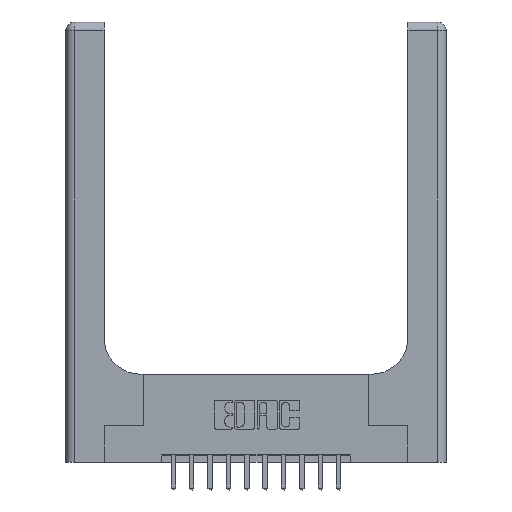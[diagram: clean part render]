
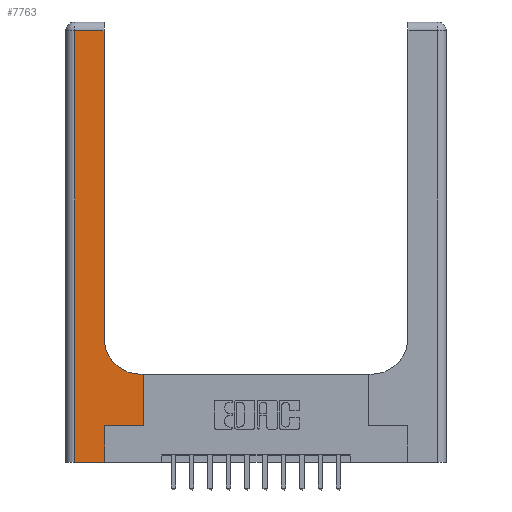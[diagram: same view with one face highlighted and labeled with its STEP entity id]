
A CAD part, top view. The second image highlights one B-rep face of the part: STEP entity #7763.
In plain terms, the highlighted planar face has unit normal (0, 0, 1).
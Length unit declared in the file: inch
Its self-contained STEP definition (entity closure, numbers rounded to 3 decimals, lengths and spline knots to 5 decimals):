
#154 = ORIENTED_EDGE ( 'NONE', *, *, #16225, .T. ) ;
#379 = EDGE_CURVE ( 'NONE', #7380, #3538, #15447, .T. ) ;
#570 = VECTOR ( 'NONE', #12872, 39.37008 ) ;
#576 = CARTESIAN_POINT ( 'NONE',  ( 0.26, 3., 0.37 ) ) ;
#1165 = VECTOR ( 'NONE', #13585, 39.37008 ) ;
#1371 = EDGE_CURVE ( 'NONE', #15486, #11015, #5670, .T. ) ;
#1570 = VERTEX_POINT ( 'NONE', #15523 ) ;
#1646 = DIRECTION ( 'NONE',  ( -1., 0., 0. ) ) ;
#1706 = VECTOR ( 'NONE', #1646, 39.37008 ) ;
#2901 = VERTEX_POINT ( 'NONE', #3424 ) ;
#3424 = CARTESIAN_POINT ( 'NONE',  ( 0.26, 0.85, 0.37 ) ) ;
#3435 = ORIENTED_EDGE ( 'NONE', *, *, #14333, .T. ) ;
#3538 = VERTEX_POINT ( 'NONE', #16037 ) ;
#3654 = CARTESIAN_POINT ( 'NONE',  ( 0.06, 0., 0.37 ) ) ;
#3705 = CARTESIAN_POINT ( 'NONE',  ( 0., 0., 0.37 ) ) ;
#3784 = EDGE_CURVE ( 'NONE', #2901, #15486, #15676, .T. ) ;
#3901 = DIRECTION ( 'NONE',  ( 1., 0., 0. ) ) ;
#4111 = VECTOR ( 'NONE', #7776, 39.37008 ) ;
#4135 = EDGE_CURVE ( 'NONE', #3538, #8264, #15314, .T. ) ;
#4285 = CARTESIAN_POINT ( 'NONE',  ( 0.26, 2.94, 0.37 ) ) ;
#4526 = ORIENTED_EDGE ( 'NONE', *, *, #379, .T. ) ;
#4615 = CARTESIAN_POINT ( 'NONE',  ( 0.51, 0.85, 0.37 ) ) ;
#4863 = AXIS2_PLACEMENT_3D ( 'NONE', #14027, #8760, #7678 ) ;
#5261 = PLANE ( 'NONE',  #4863 ) ;
#5432 = EDGE_CURVE ( 'NONE', #1570, #2901, #13335, .T. ) ;
#5670 = LINE ( 'NONE', #10921, #1165 ) ;
#7380 = VERTEX_POINT ( 'NONE', #12866 ) ;
#7503 = FACE_OUTER_BOUND ( 'NONE', #15960, .T. ) ;
#7634 = VECTOR ( 'NONE', #13767, 39.37008 ) ;
#7678 = DIRECTION ( 'NONE',  ( -1., 0., 0. ) ) ;
#7763 = ADVANCED_FACE ( 'NONE', ( #7503 ), #5261, .F. ) ;
#7776 = DIRECTION ( 'NONE',  ( 0., 1., 0. ) ) ;
#8211 = DIRECTION ( 'NONE',  ( 0., 1., 0. ) ) ;
#8264 = VERTEX_POINT ( 'NONE', #15177 ) ;
#8537 = AXIS2_PLACEMENT_3D ( 'NONE', #4615, #9543, #13474 ) ;
#8679 = LINE ( 'NONE', #10003, #7634 ) ;
#8732 = ORIENTED_EDGE ( 'NONE', *, *, #3784, .T. ) ;
#8760 = DIRECTION ( 'NONE',  ( 0., 0., -1. ) ) ;
#9213 = ORIENTED_EDGE ( 'NONE', *, *, #10492, .T. ) ;
#9543 = DIRECTION ( 'NONE',  ( 0., 0., -1. ) ) ;
#9678 = ORIENTED_EDGE ( 'NONE', *, *, #5432, .T. ) ;
#9757 = ORIENTED_EDGE ( 'NONE', *, *, #4135, .T. ) ;
#10003 = CARTESIAN_POINT ( 'NONE',  ( 0.06, 3., 0.37 ) ) ;
#10386 = ORIENTED_EDGE ( 'NONE', *, *, #14854, .T. ) ;
#10406 = CARTESIAN_POINT ( 'NONE',  ( 0.265, 0.25, 0.37 ) ) ;
#10492 = EDGE_CURVE ( 'NONE', #14271, #7380, #10614, .T. ) ;
#10614 = LINE ( 'NONE', #15739, #570 ) ;
#10623 = ORIENTED_EDGE ( 'NONE', *, *, #1371, .T. ) ;
#10921 = CARTESIAN_POINT ( 'NONE',  ( 0., 2.94, 0.37 ) ) ;
#11015 = VERTEX_POINT ( 'NONE', #15548 ) ;
#11485 = LINE ( 'NONE', #3705, #16135 ) ;
#11856 = VECTOR ( 'NONE', #3901, 39.37008 ) ;
#12397 = CARTESIAN_POINT ( 'NONE',  ( 0.265, 0., 0.37 ) ) ;
#12612 = CARTESIAN_POINT ( 'NONE',  ( 0.26, 0.6, 0.37 ) ) ;
#12866 = CARTESIAN_POINT ( 'NONE',  ( 0.265, 0.25, 0.37 ) ) ;
#12872 = DIRECTION ( 'NONE',  ( 0., 1., 0. ) ) ;
#13335 = CIRCLE ( 'NONE', #8537, 0.25 ) ;
#13474 = DIRECTION ( 'NONE',  ( 1., 0., 0. ) ) ;
#13585 = DIRECTION ( 'NONE',  ( -1., 0., 0. ) ) ;
#13767 = DIRECTION ( 'NONE',  ( 0., -1., 0. ) ) ;
#13865 = LINE ( 'NONE', #12612, #1706 ) ;
#14027 = CARTESIAN_POINT ( 'NONE',  ( 0., 3., 0.37 ) ) ;
#14123 = CARTESIAN_POINT ( 'NONE',  ( 0.528, 0.25, 0.37 ) ) ;
#14271 = VERTEX_POINT ( 'NONE', #12397 ) ;
#14333 = EDGE_CURVE ( 'NONE', #15175, #14271, #11485, .T. ) ;
#14854 = EDGE_CURVE ( 'NONE', #8264, #1570, #13865, .T. ) ;
#15018 = VECTOR ( 'NONE', #8211, 39.37008 ) ;
#15175 = VERTEX_POINT ( 'NONE', #3654 ) ;
#15177 = CARTESIAN_POINT ( 'NONE',  ( 0.528, 0.6, 0.37 ) ) ;
#15314 = LINE ( 'NONE', #14123, #4111 ) ;
#15447 = LINE ( 'NONE', #10406, #11856 ) ;
#15486 = VERTEX_POINT ( 'NONE', #4285 ) ;
#15523 = CARTESIAN_POINT ( 'NONE',  ( 0.51, 0.6, 0.37 ) ) ;
#15548 = CARTESIAN_POINT ( 'NONE',  ( 0.06, 2.94, 0.37 ) ) ;
#15676 = LINE ( 'NONE', #576, #15018 ) ;
#15739 = CARTESIAN_POINT ( 'NONE',  ( 0.265, 0., 0.37 ) ) ;
#15960 = EDGE_LOOP ( 'NONE', ( #8732, #10623, #154, #3435, #9213, #4526, #9757, #10386, #9678 ) ) ;
#16037 = CARTESIAN_POINT ( 'NONE',  ( 0.528, 0.25, 0.37 ) ) ;
#16135 = VECTOR ( 'NONE', #16342, 39.37008 ) ;
#16225 = EDGE_CURVE ( 'NONE', #11015, #15175, #8679, .T. ) ;
#16342 = DIRECTION ( 'NONE',  ( 1., 0., 0. ) ) ;
